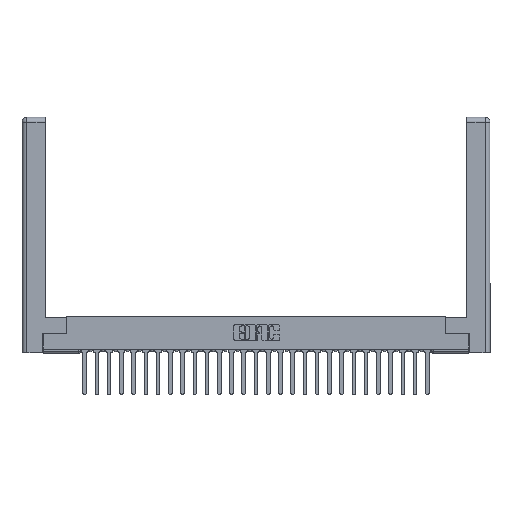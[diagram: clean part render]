
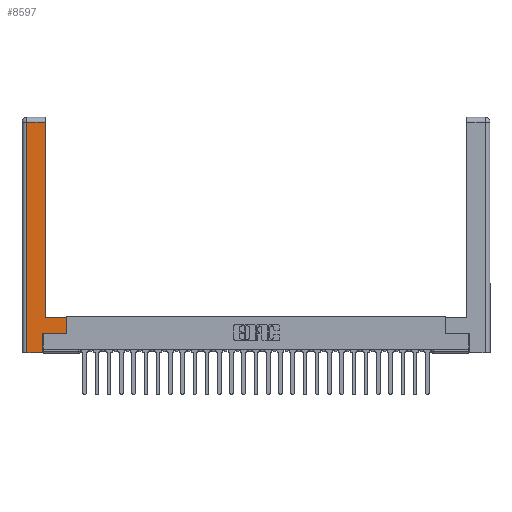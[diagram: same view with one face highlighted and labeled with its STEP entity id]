
A CAD part, top view. The second image highlights one B-rep face of the part: STEP entity #8597.
In plain terms, the highlighted planar face has unit normal (0, 0, 1).
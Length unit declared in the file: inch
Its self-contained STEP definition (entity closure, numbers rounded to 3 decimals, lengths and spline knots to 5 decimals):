
#47 = ORIENTED_EDGE ( 'NONE', *, *, #16503, .T. ) ;
#667 = ORIENTED_EDGE ( 'NONE', *, *, #16128, .T. ) ;
#1124 = DIRECTION ( 'NONE',  ( 1., 0., 0. ) ) ;
#1169 = DIRECTION ( 'NONE',  ( -1., 0., 0. ) ) ;
#1642 = FACE_OUTER_BOUND ( 'NONE', #21482, .T. ) ;
#1670 = VERTEX_POINT ( 'NONE', #22280 ) ;
#1867 = CARTESIAN_POINT ( 'NONE',  ( 0.295, 0.45, 0. ) ) ;
#2152 = EDGE_CURVE ( 'NONE', #9434, #25840, #25727, .T. ) ;
#2416 = VERTEX_POINT ( 'NONE', #4702 ) ;
#3073 = ORIENTED_EDGE ( 'NONE', *, *, #21571, .T. ) ;
#3590 = VECTOR ( 'NONE', #21378, 39.37008 ) ;
#4215 = DIRECTION ( 'NONE',  ( 0., 0., -1. ) ) ;
#4702 = CARTESIAN_POINT ( 'NONE',  ( 0.565, 0.45, 0. ) ) ;
#5038 = EDGE_CURVE ( 'NONE', #21764, #29046, #15094, .T. ) ;
#5606 = VECTOR ( 'NONE', #14976, 39.37008 ) ;
#6297 = CARTESIAN_POINT ( 'NONE',  ( 0.265, 0., 0. ) ) ;
#6629 = ORIENTED_EDGE ( 'NONE', *, *, #5038, .T. ) ;
#7420 = LINE ( 'NONE', #28347, #3590 ) ;
#8205 = ORIENTED_EDGE ( 'NONE', *, *, #2152, .T. ) ;
#8597 = ADVANCED_FACE ( 'NONE', ( #1642 ), #20153, .F. ) ;
#8736 = ORIENTED_EDGE ( 'NONE', *, *, #18069, .T. ) ;
#8744 = LINE ( 'NONE', #11162, #22671 ) ;
#9434 = VERTEX_POINT ( 'NONE', #1867 ) ;
#9601 = CARTESIAN_POINT ( 'NONE',  ( 0.565, 0.45, 0. ) ) ;
#9726 = CARTESIAN_POINT ( 'NONE',  ( 0.295, 0.45, 0. ) ) ;
#11162 = CARTESIAN_POINT ( 'NONE',  ( 0.565, 0.245, 0. ) ) ;
#11685 = LINE ( 'NONE', #9726, #15710 ) ;
#12171 = VECTOR ( 'NONE', #1169, 39.37008 ) ;
#12808 = EDGE_CURVE ( 'NONE', #25840, #1670, #28674, .T. ) ;
#14787 = CARTESIAN_POINT ( 'NONE',  ( 0.265, 0., 0. ) ) ;
#14976 = DIRECTION ( 'NONE',  ( 0., -1., 0. ) ) ;
#15094 = LINE ( 'NONE', #14787, #18042 ) ;
#15557 = VECTOR ( 'NONE', #23153, 39.37008 ) ;
#15638 = EDGE_CURVE ( 'NONE', #22676, #2416, #17042, .T. ) ;
#15710 = VECTOR ( 'NONE', #23373, 39.37008 ) ;
#16128 = EDGE_CURVE ( 'NONE', #2416, #9434, #11685, .T. ) ;
#16172 = ORIENTED_EDGE ( 'NONE', *, *, #12808, .T. ) ;
#16503 = EDGE_CURVE ( 'NONE', #29046, #29952, #7420, .T. ) ;
#17042 = LINE ( 'NONE', #9601, #18107 ) ;
#17245 = CARTESIAN_POINT ( 'NONE',  ( 0.565, 0.245, 0. ) ) ;
#18015 = ORIENTED_EDGE ( 'NONE', *, *, #15638, .T. ) ;
#18042 = VECTOR ( 'NONE', #1124, 39.37008 ) ;
#18069 = EDGE_CURVE ( 'NONE', #1670, #21764, #26519, .T. ) ;
#18107 = VECTOR ( 'NONE', #19309, 39.37008 ) ;
#18511 = AXIS2_PLACEMENT_3D ( 'NONE', #29438, #4215, #27154 ) ;
#19309 = DIRECTION ( 'NONE',  ( 0., 1., 0. ) ) ;
#19696 = CARTESIAN_POINT ( 'NONE',  ( 0.0615, 2.94, 0. ) ) ;
#20153 = PLANE ( 'NONE',  #18511 ) ;
#20336 = CARTESIAN_POINT ( 'NONE',  ( 0.295, 2.94, 0. ) ) ;
#21335 = CARTESIAN_POINT ( 'NONE',  ( 0.295, 3., 0. ) ) ;
#21378 = DIRECTION ( 'NONE',  ( 0., 1., 0. ) ) ;
#21482 = EDGE_LOOP ( 'NONE', ( #8205, #16172, #8736, #6629, #47, #3073, #18015, #667 ) ) ;
#21571 = EDGE_CURVE ( 'NONE', #29952, #22676, #8744, .T. ) ;
#21764 = VERTEX_POINT ( 'NONE', #24472 ) ;
#22280 = CARTESIAN_POINT ( 'NONE',  ( 0.0615, 2.94, 0. ) ) ;
#22671 = VECTOR ( 'NONE', #29389, 39.37008 ) ;
#22676 = VERTEX_POINT ( 'NONE', #17245 ) ;
#22743 = CARTESIAN_POINT ( 'NONE',  ( 0.265, 0.245, 0. ) ) ;
#23153 = DIRECTION ( 'NONE',  ( 0., 1., 0. ) ) ;
#23373 = DIRECTION ( 'NONE',  ( -1., 0., 0. ) ) ;
#24472 = CARTESIAN_POINT ( 'NONE',  ( 0.0615, 0., 0. ) ) ;
#25727 = LINE ( 'NONE', #21335, #15557 ) ;
#25840 = VERTEX_POINT ( 'NONE', #20336 ) ;
#26519 = LINE ( 'NONE', #28662, #5606 ) ;
#27154 = DIRECTION ( 'NONE',  ( -1., 0., 0. ) ) ;
#28347 = CARTESIAN_POINT ( 'NONE',  ( 0.265, 0.245, 0. ) ) ;
#28662 = CARTESIAN_POINT ( 'NONE',  ( 0.0615, 0., 0. ) ) ;
#28674 = LINE ( 'NONE', #19696, #12171 ) ;
#29046 = VERTEX_POINT ( 'NONE', #6297 ) ;
#29389 = DIRECTION ( 'NONE',  ( 1., 0., 0. ) ) ;
#29438 = CARTESIAN_POINT ( 'NONE',  ( 0., 0., 0. ) ) ;
#29952 = VERTEX_POINT ( 'NONE', #22743 ) ;
